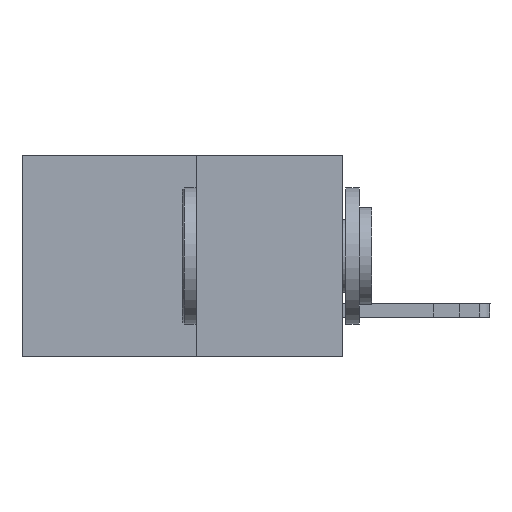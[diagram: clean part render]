
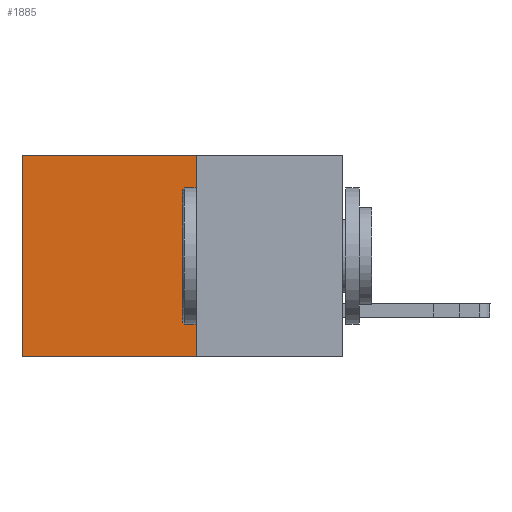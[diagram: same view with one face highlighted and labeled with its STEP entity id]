
A CAD part, left-side view. The second image highlights one B-rep face of the part: STEP entity #1885.
In plain terms, the highlighted planar face has unit normal (-1, 0, 0).
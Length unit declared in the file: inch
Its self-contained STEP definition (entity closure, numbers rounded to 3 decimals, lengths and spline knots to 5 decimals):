
#244 = CARTESIAN_POINT ( 'NONE',  ( 0.277, 0.27, 0. ) ) ;
#465 = EDGE_CURVE ( 'NONE', #9573, #6492, #19295, .T. ) ;
#697 = AXIS2_PLACEMENT_3D ( 'NONE', #4280, #1294, #10015 ) ;
#1294 = DIRECTION ( 'NONE',  ( 1., 0., 0. ) ) ;
#1642 = EDGE_CURVE ( 'NONE', #4604, #9708, #7177, .T. ) ;
#1885 = ADVANCED_FACE ( 'NONE', ( #14594 ), #19124, .F. ) ;
#2388 = CARTESIAN_POINT ( 'NONE',  ( 0.277, 0.27, -0.37 ) ) ;
#2738 = CARTESIAN_POINT ( 'NONE',  ( 0.277, 0.59, 0. ) ) ;
#2977 = ORIENTED_EDGE ( 'NONE', *, *, #13695, .F. ) ;
#3342 = VECTOR ( 'NONE', #10169, 39.37008 ) ;
#3796 = DIRECTION ( 'NONE',  ( 0., 0., -1. ) ) ;
#4280 = CARTESIAN_POINT ( 'NONE',  ( 0.277, 0.27, -0.37 ) ) ;
#4604 = VERTEX_POINT ( 'NONE', #2388 ) ;
#5201 = VECTOR ( 'NONE', #3796, 39.37008 ) ;
#6492 = VERTEX_POINT ( 'NONE', #2738 ) ;
#6882 = CARTESIAN_POINT ( 'NONE',  ( 0.277, 0.59, -0.37 ) ) ;
#7177 = LINE ( 'NONE', #15621, #10811 ) ;
#7475 = LINE ( 'NONE', #17663, #3342 ) ;
#9219 = DIRECTION ( 'NONE',  ( 0., 1., 0. ) ) ;
#9573 = VERTEX_POINT ( 'NONE', #17286 ) ;
#9708 = VERTEX_POINT ( 'NONE', #10555 ) ;
#10015 = DIRECTION ( 'NONE',  ( 0., 0., -1. ) ) ;
#10169 = DIRECTION ( 'NONE',  ( 0., 0., -1. ) ) ;
#10555 = CARTESIAN_POINT ( 'NONE',  ( 0.277, 0.59, -0.37 ) ) ;
#10811 = VECTOR ( 'NONE', #17033, 39.37008 ) ;
#11013 = EDGE_CURVE ( 'NONE', #6492, #9708, #17432, .T. ) ;
#11872 = ORIENTED_EDGE ( 'NONE', *, *, #11013, .T. ) ;
#13695 = EDGE_CURVE ( 'NONE', #9573, #4604, #7475, .T. ) ;
#14594 = FACE_OUTER_BOUND ( 'NONE', #15273, .T. ) ;
#15273 = EDGE_LOOP ( 'NONE', ( #11872, #18329, #2977, #19646 ) ) ;
#15304 = VECTOR ( 'NONE', #9219, 39.37008 ) ;
#15621 = CARTESIAN_POINT ( 'NONE',  ( 0.277, 0.27, -0.37 ) ) ;
#17033 = DIRECTION ( 'NONE',  ( 0., 1., 0. ) ) ;
#17286 = CARTESIAN_POINT ( 'NONE',  ( 0.277, 0.27, 0. ) ) ;
#17432 = LINE ( 'NONE', #6882, #5201 ) ;
#17663 = CARTESIAN_POINT ( 'NONE',  ( 0.277, 0.27, -0.37 ) ) ;
#18329 = ORIENTED_EDGE ( 'NONE', *, *, #1642, .F. ) ;
#19124 = PLANE ( 'NONE',  #697 ) ;
#19295 = LINE ( 'NONE', #244, #15304 ) ;
#19646 = ORIENTED_EDGE ( 'NONE', *, *, #465, .T. ) ;
